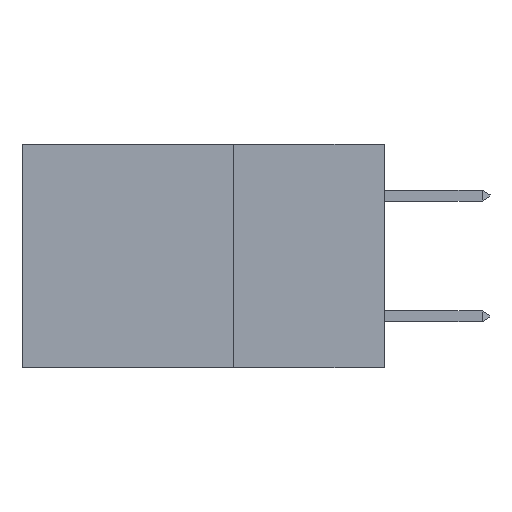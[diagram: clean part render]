
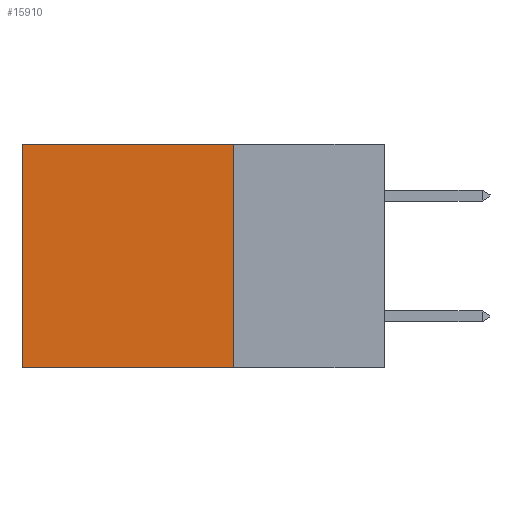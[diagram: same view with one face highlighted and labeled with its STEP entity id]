
A CAD part, left-side view. The second image highlights one B-rep face of the part: STEP entity #15910.
In plain terms, the highlighted planar face has unit normal (-1, 0, 0).
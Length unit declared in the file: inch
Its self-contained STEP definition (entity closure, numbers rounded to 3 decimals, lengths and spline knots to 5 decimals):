
#259 = VERTEX_POINT ( 'NONE', #16162 ) ;
#319 = VECTOR ( 'NONE', #16231, 39.37008 ) ;
#1303 = VECTOR ( 'NONE', #9957, 39.37008 ) ;
#1620 = EDGE_CURVE ( 'NONE', #259, #27219, #22131, .T. ) ;
#2741 = DIRECTION ( 'NONE',  ( 1., 0., 0. ) ) ;
#4413 = FACE_OUTER_BOUND ( 'NONE', #5341, .T. ) ;
#5341 = EDGE_LOOP ( 'NONE', ( #15857, #11373, #12904, #21312 ) ) ;
#5680 = EDGE_CURVE ( 'NONE', #7713, #10429, #23176, .T. ) ;
#6382 = PLANE ( 'NONE',  #20830 ) ;
#7713 = VERTEX_POINT ( 'NONE', #24746 ) ;
#7922 = VECTOR ( 'NONE', #11214, 39.37008 ) ;
#8384 = CARTESIAN_POINT ( 'NONE',  ( 0.2875, 0.25, -0.37 ) ) ;
#8917 = EDGE_CURVE ( 'NONE', #27219, #10429, #30652, .T. ) ;
#9957 = DIRECTION ( 'NONE',  ( 0., 1., 0. ) ) ;
#10328 = DIRECTION ( 'NONE',  ( 0., 0., -1. ) ) ;
#10429 = VERTEX_POINT ( 'NONE', #11759 ) ;
#11196 = CARTESIAN_POINT ( 'NONE',  ( 0.2875, 0.25, 0. ) ) ;
#11214 = DIRECTION ( 'NONE',  ( 0., 1., 0. ) ) ;
#11373 = ORIENTED_EDGE ( 'NONE', *, *, #5680, .F. ) ;
#11759 = CARTESIAN_POINT ( 'NONE',  ( 0.2875, 0.6, -0.37 ) ) ;
#12757 = CARTESIAN_POINT ( 'NONE',  ( 0.2875, 0.6, 0. ) ) ;
#12904 = ORIENTED_EDGE ( 'NONE', *, *, #14022, .F. ) ;
#13323 = DIRECTION ( 'NONE',  ( 0., 0., -1. ) ) ;
#14022 = EDGE_CURVE ( 'NONE', #259, #7713, #31455, .T. ) ;
#15857 = ORIENTED_EDGE ( 'NONE', *, *, #8917, .T. ) ;
#15910 = ADVANCED_FACE ( 'NONE', ( #4413 ), #6382, .F. ) ;
#16162 = CARTESIAN_POINT ( 'NONE',  ( 0.2875, 0.25, 0. ) ) ;
#16231 = DIRECTION ( 'NONE',  ( 0., 0., -1. ) ) ;
#18301 = VECTOR ( 'NONE', #13323, 39.37008 ) ;
#20830 = AXIS2_PLACEMENT_3D ( 'NONE', #22242, #2741, #10328 ) ;
#21312 = ORIENTED_EDGE ( 'NONE', *, *, #1620, .T. ) ;
#22131 = LINE ( 'NONE', #23883, #7922 ) ;
#22242 = CARTESIAN_POINT ( 'NONE',  ( 0.2875, 0.25, 0. ) ) ;
#23176 = LINE ( 'NONE', #8384, #1303 ) ;
#23883 = CARTESIAN_POINT ( 'NONE',  ( 0.2875, 0.25, 0. ) ) ;
#24430 = CARTESIAN_POINT ( 'NONE',  ( 0.2875, 0.6, 0. ) ) ;
#24746 = CARTESIAN_POINT ( 'NONE',  ( 0.2875, 0.25, -0.37 ) ) ;
#27219 = VERTEX_POINT ( 'NONE', #24430 ) ;
#30652 = LINE ( 'NONE', #12757, #18301 ) ;
#31455 = LINE ( 'NONE', #11196, #319 ) ;
